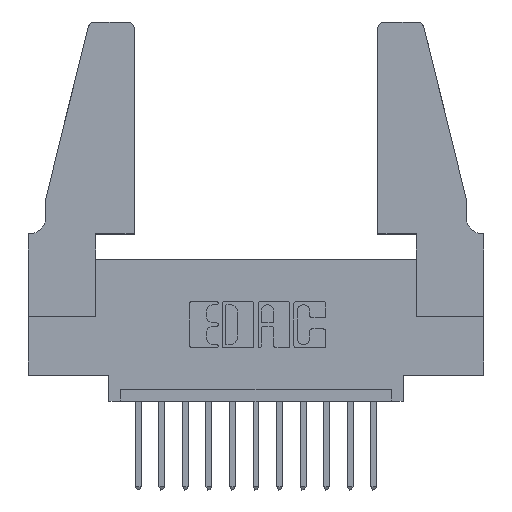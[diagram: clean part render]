
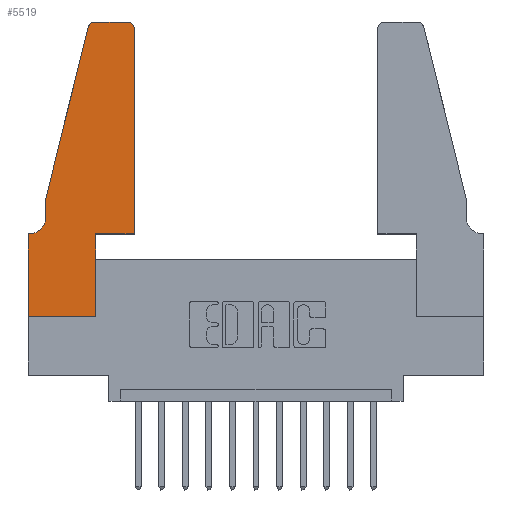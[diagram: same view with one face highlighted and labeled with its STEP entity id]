
A CAD part, top view. The second image highlights one B-rep face of the part: STEP entity #5519.
In plain terms, the highlighted planar face has unit normal (0, 0, 1).
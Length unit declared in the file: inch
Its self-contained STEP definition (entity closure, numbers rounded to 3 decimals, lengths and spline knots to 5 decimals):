
#49 = DIRECTION ( 'NONE',  ( -1., 0., 0. ) ) ;
#124 = LINE ( 'NONE', #4427, #13336 ) ;
#172 = AXIS2_PLACEMENT_3D ( 'NONE', #9094, #4577, #2382 ) ;
#220 = EDGE_CURVE ( 'NONE', #10010, #10001, #1471, .T. ) ;
#283 = VERTEX_POINT ( 'NONE', #5900 ) ;
#385 = CARTESIAN_POINT ( 'NONE',  ( 0.0755, 0.35, 0.37 ) ) ;
#478 = EDGE_LOOP ( 'NONE', ( #6342, #13242, #5266, #2663, #11805, #8936, #6406, #12977, #5428, #11306, #3025, #11715 ) ) ;
#579 = AXIS2_PLACEMENT_3D ( 'NONE', #1144, #5752, #10385 ) ;
#583 = VERTEX_POINT ( 'NONE', #3706 ) ;
#698 = VERTEX_POINT ( 'NONE', #8384 ) ;
#878 = DIRECTION ( 'NONE',  ( 1., 0., 0. ) ) ;
#1110 = VERTEX_POINT ( 'NONE', #4820 ) ;
#1144 = CARTESIAN_POINT ( 'NONE',  ( 0.4205, 1.22, 0.37 ) ) ;
#1403 = LINE ( 'NONE', #7578, #5359 ) ;
#1471 = LINE ( 'NONE', #3445, #8074 ) ;
#2264 = DIRECTION ( 'NONE',  ( 0., 0., 1. ) ) ;
#2382 = DIRECTION ( 'NONE',  ( 1., 0., 0. ) ) ;
#2655 = EDGE_CURVE ( 'NONE', #10001, #9040, #4980, .T. ) ;
#2663 = ORIENTED_EDGE ( 'NONE', *, *, #7770, .T. ) ;
#2767 = DIRECTION ( 'NONE',  ( 0., 1., 0. ) ) ;
#2879 = VERTEX_POINT ( 'NONE', #10402 ) ;
#3019 = CARTESIAN_POINT ( 'NONE',  ( 0.2865, 0.35, 0.37 ) ) ;
#3025 = ORIENTED_EDGE ( 'NONE', *, *, #10480, .T. ) ;
#3110 = CARTESIAN_POINT ( 'NONE',  ( 0.25487, 1.22718, 0.37 ) ) ;
#3445 = CARTESIAN_POINT ( 'NONE',  ( 0.2605, 1.25, 0.37 ) ) ;
#3706 = CARTESIAN_POINT ( 'NONE',  ( 0., 0.35, 0.37 ) ) ;
#3867 = VECTOR ( 'NONE', #7223, 39.37008 ) ;
#3951 = DIRECTION ( 'NONE',  ( 0., -1., 0. ) ) ;
#4258 = VECTOR ( 'NONE', #7286, 39.37008 ) ;
#4355 = DIRECTION ( 'NONE',  ( -0.239, -0.971, 0. ) ) ;
#4427 = CARTESIAN_POINT ( 'NONE',  ( 0.0755, 0.5, 0.37 ) ) ;
#4577 = DIRECTION ( 'NONE',  ( 0., 0., 1. ) ) ;
#4676 = PLANE ( 'NONE',  #172 ) ;
#4720 = VERTEX_POINT ( 'NONE', #9474 ) ;
#4777 = AXIS2_PLACEMENT_3D ( 'NONE', #13078, #6271, #9548 ) ;
#4820 = CARTESIAN_POINT ( 'NONE',  ( 0.4505, 0.35, 0.37 ) ) ;
#4862 = CIRCLE ( 'NONE', #579, 0.03 ) ;
#4946 = LINE ( 'NONE', #9452, #3867 ) ;
#4980 = CIRCLE ( 'NONE', #7043, 0.03 ) ;
#4984 = DIRECTION ( 'NONE',  ( 1., 0., 0. ) ) ;
#5266 = ORIENTED_EDGE ( 'NONE', *, *, #11796, .T. ) ;
#5285 = CARTESIAN_POINT ( 'NONE',  ( 0.284, 1.25, 0.37 ) ) ;
#5359 = VECTOR ( 'NONE', #878, 39.37008 ) ;
#5428 = ORIENTED_EDGE ( 'NONE', *, *, #7837, .T. ) ;
#5519 = ADVANCED_FACE ( 'NONE', ( #9901 ), #4676, .T. ) ;
#5752 = DIRECTION ( 'NONE',  ( 0., 0., 1. ) ) ;
#5837 = EDGE_CURVE ( 'NONE', #4720, #6826, #10213, .T. ) ;
#5892 = VERTEX_POINT ( 'NONE', #11109 ) ;
#5900 = CARTESIAN_POINT ( 'NONE',  ( 0., 0., 0.37 ) ) ;
#6271 = DIRECTION ( 'NONE',  ( 0., 0., -1. ) ) ;
#6342 = ORIENTED_EDGE ( 'NONE', *, *, #220, .T. ) ;
#6406 = ORIENTED_EDGE ( 'NONE', *, *, #11582, .T. ) ;
#6618 = EDGE_CURVE ( 'NONE', #2879, #10010, #4862, .T. ) ;
#6637 = VECTOR ( 'NONE', #3951, 39.37008 ) ;
#6667 = CARTESIAN_POINT ( 'NONE',  ( 0.0755, 0.5, 0.37 ) ) ;
#6826 = VERTEX_POINT ( 'NONE', #12691 ) ;
#7043 = AXIS2_PLACEMENT_3D ( 'NONE', #9205, #2264, #14785 ) ;
#7206 = CARTESIAN_POINT ( 'NONE',  ( 0.4505, 0.35, 0.37 ) ) ;
#7223 = DIRECTION ( 'NONE',  ( 0., 1., 0. ) ) ;
#7286 = DIRECTION ( 'NONE',  ( -1., 0., 0. ) ) ;
#7564 = CARTESIAN_POINT ( 'NONE',  ( 0.4205, 1.25, 0.37 ) ) ;
#7578 = CARTESIAN_POINT ( 'NONE',  ( 0., 0., 0.37 ) ) ;
#7662 = VECTOR ( 'NONE', #4984, 39.37008 ) ;
#7770 = EDGE_CURVE ( 'NONE', #5892, #4720, #124, .T. ) ;
#7837 = EDGE_CURVE ( 'NONE', #698, #14277, #4946, .T. ) ;
#8074 = VECTOR ( 'NONE', #49, 39.37008 ) ;
#8384 = CARTESIAN_POINT ( 'NONE',  ( 0.2865, 0., 0.37 ) ) ;
#8416 = CARTESIAN_POINT ( 'NONE',  ( 0.4505, 0.35, 0.37 ) ) ;
#8720 = LINE ( 'NONE', #8416, #7662 ) ;
#8936 = ORIENTED_EDGE ( 'NONE', *, *, #12805, .T. ) ;
#9040 = VERTEX_POINT ( 'NONE', #3110 ) ;
#9094 = CARTESIAN_POINT ( 'NONE',  ( 0., 0.35, 0.37 ) ) ;
#9205 = CARTESIAN_POINT ( 'NONE',  ( 0.284, 1.22, 0.37 ) ) ;
#9452 = CARTESIAN_POINT ( 'NONE',  ( 0.2865, 0.35, 0.37 ) ) ;
#9474 = CARTESIAN_POINT ( 'NONE',  ( 0.0755, 0.42, 0.37 ) ) ;
#9548 = DIRECTION ( 'NONE',  ( -1., 0., 0. ) ) ;
#9901 = FACE_OUTER_BOUND ( 'NONE', #478, .T. ) ;
#10001 = VERTEX_POINT ( 'NONE', #5285 ) ;
#10010 = VERTEX_POINT ( 'NONE', #7564 ) ;
#10213 = CIRCLE ( 'NONE', #4777, 0.07 ) ;
#10385 = DIRECTION ( 'NONE',  ( 1., 0., 0. ) ) ;
#10402 = CARTESIAN_POINT ( 'NONE',  ( 0.4505, 1.22, 0.37 ) ) ;
#10480 = EDGE_CURVE ( 'NONE', #1110, #2879, #11824, .T. ) ;
#10889 = VECTOR ( 'NONE', #4355, 39.37008 ) ;
#11053 = LINE ( 'NONE', #385, #4258 ) ;
#11109 = CARTESIAN_POINT ( 'NONE',  ( 0.0755, 0.5, 0.37 ) ) ;
#11306 = ORIENTED_EDGE ( 'NONE', *, *, #12832, .T. ) ;
#11582 = EDGE_CURVE ( 'NONE', #583, #283, #14474, .T. ) ;
#11715 = ORIENTED_EDGE ( 'NONE', *, *, #6618, .T. ) ;
#11796 = EDGE_CURVE ( 'NONE', #9040, #5892, #12323, .T. ) ;
#11805 = ORIENTED_EDGE ( 'NONE', *, *, #5837, .T. ) ;
#11824 = LINE ( 'NONE', #7206, #13759 ) ;
#11939 = EDGE_CURVE ( 'NONE', #283, #698, #1403, .T. ) ;
#12103 = CARTESIAN_POINT ( 'NONE',  ( 0., 0., 0.37 ) ) ;
#12271 = DIRECTION ( 'NONE',  ( 0., -1., 0. ) ) ;
#12323 = LINE ( 'NONE', #6667, #10889 ) ;
#12691 = CARTESIAN_POINT ( 'NONE',  ( 0.0055, 0.35, 0.37 ) ) ;
#12805 = EDGE_CURVE ( 'NONE', #6826, #583, #11053, .T. ) ;
#12832 = EDGE_CURVE ( 'NONE', #14277, #1110, #8720, .T. ) ;
#12977 = ORIENTED_EDGE ( 'NONE', *, *, #11939, .T. ) ;
#13078 = CARTESIAN_POINT ( 'NONE',  ( 0.0055, 0.42, 0.37 ) ) ;
#13242 = ORIENTED_EDGE ( 'NONE', *, *, #2655, .T. ) ;
#13336 = VECTOR ( 'NONE', #12271, 39.37008 ) ;
#13759 = VECTOR ( 'NONE', #2767, 39.37008 ) ;
#14277 = VERTEX_POINT ( 'NONE', #3019 ) ;
#14474 = LINE ( 'NONE', #12103, #6637 ) ;
#14785 = DIRECTION ( 'NONE',  ( 1., 0., 0. ) ) ;
